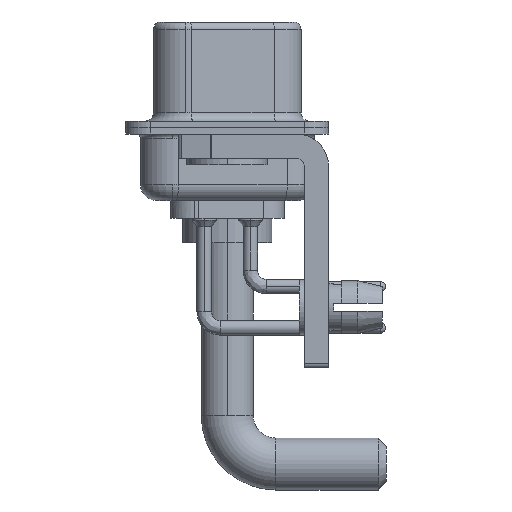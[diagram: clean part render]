
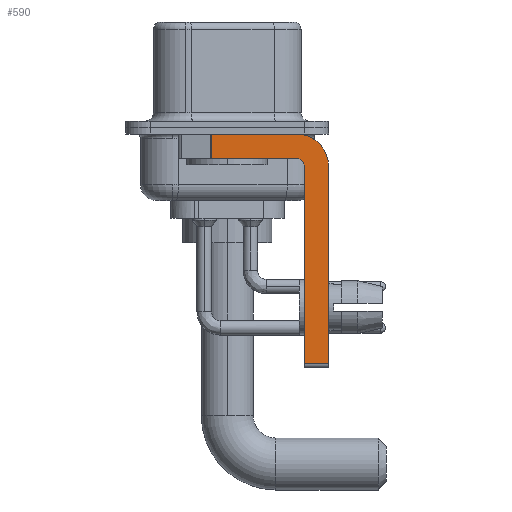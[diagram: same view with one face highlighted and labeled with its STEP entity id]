
A CAD part, left-side view. The second image highlights one B-rep face of the part: STEP entity #590.
In plain terms, the highlighted planar face has unit normal (-1, 0, 0).
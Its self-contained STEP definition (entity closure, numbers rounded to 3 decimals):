
#542 = VECTOR ( 'NONE', #23690, 1000. ) ;
#590 = ADVANCED_FACE ( 'NONE', ( #19994 ), #11389, .F. ) ;
#682 = VERTEX_POINT ( 'NONE', #23240 ) ;
#734 = LINE ( 'NONE', #13457, #12163 ) ;
#1258 = VERTEX_POINT ( 'NONE', #10749 ) ;
#1334 = ORIENTED_EDGE ( 'NONE', *, *, #7442, .T. ) ;
#1344 = VERTEX_POINT ( 'NONE', #19079 ) ;
#1639 = EDGE_CURVE ( 'NONE', #10639, #682, #2580, .T. ) ;
#1990 = DIRECTION ( 'NONE',  ( -1., 0., 0. ) ) ;
#2530 = CARTESIAN_POINT ( 'NONE',  ( -2.9, -4.25, -14.55 ) ) ;
#2580 = CIRCLE ( 'NONE', #28166, 0.5 ) ;
#2780 = CARTESIAN_POINT ( 'NONE',  ( -2.9, -4.75, -14.55 ) ) ;
#3087 = DIRECTION ( 'NONE',  ( 0., 0., -1. ) ) ;
#3308 = VECTOR ( 'NONE', #16369, 1000. ) ;
#3680 = CARTESIAN_POINT ( 'NONE',  ( -2.9, -4.25, -1.9 ) ) ;
#3988 = EDGE_CURVE ( 'NONE', #1344, #25224, #22690, .T. ) ;
#4282 = LINE ( 'NONE', #21493, #17298 ) ;
#4372 = VERTEX_POINT ( 'NONE', #2780 ) ;
#4803 = CARTESIAN_POINT ( 'NONE',  ( -2.9, 3., -0.4 ) ) ;
#5787 = CIRCLE ( 'NONE', #21787, 2. ) ;
#7180 = EDGE_CURVE ( 'NONE', #682, #1258, #21429, .T. ) ;
#7442 = EDGE_CURVE ( 'NONE', #1344, #1258, #11670, .T. ) ;
#9121 = DIRECTION ( 'NONE',  ( 0., -1., 0. ) ) ;
#9535 = LINE ( 'NONE', #2530, #22934 ) ;
#10587 = CARTESIAN_POINT ( 'NONE',  ( -2.9, -4.25, -2.4 ) ) ;
#10639 = VERTEX_POINT ( 'NONE', #20645 ) ;
#10749 = CARTESIAN_POINT ( 'NONE',  ( -2.9, 0.978, -1.9 ) ) ;
#10981 = EDGE_CURVE ( 'NONE', #4372, #15280, #9535, .T. ) ;
#11389 = PLANE ( 'NONE',  #14396 ) ;
#11574 = CARTESIAN_POINT ( 'NONE',  ( -2.9, -4.25, -2.4 ) ) ;
#11670 = LINE ( 'NONE', #27244, #3308 ) ;
#12163 = VECTOR ( 'NONE', #20488, 1000. ) ;
#13457 = CARTESIAN_POINT ( 'NONE',  ( -2.9, -6.25, -2.4 ) ) ;
#13655 = VECTOR ( 'NONE', #26689, 1000. ) ;
#14396 = AXIS2_PLACEMENT_3D ( 'NONE', #15812, #26562, #3087 ) ;
#15280 = VERTEX_POINT ( 'NONE', #27460 ) ;
#15756 = ORIENTED_EDGE ( 'NONE', *, *, #1639, .F. ) ;
#15812 = CARTESIAN_POINT ( 'NONE',  ( -2.9, -4.25, -2.4 ) ) ;
#16369 = DIRECTION ( 'NONE',  ( 0., 0., -1. ) ) ;
#16483 = EDGE_CURVE ( 'NONE', #27638, #15280, #734, .T. ) ;
#16925 = EDGE_CURVE ( 'NONE', #25224, #27638, #5787, .T. ) ;
#17298 = VECTOR ( 'NONE', #25756, 1000. ) ;
#17364 = EDGE_LOOP ( 'NONE', ( #22047, #1334, #21734, #15756, #26348, #23552, #20946, #27428 ) ) ;
#18822 = CARTESIAN_POINT ( 'NONE',  ( -2.9, -6.25, -2.4 ) ) ;
#19079 = CARTESIAN_POINT ( 'NONE',  ( -2.9, 0.978, -0.4 ) ) ;
#19994 = FACE_OUTER_BOUND ( 'NONE', #17364, .T. ) ;
#20488 = DIRECTION ( 'NONE',  ( 0., 0., -1. ) ) ;
#20645 = CARTESIAN_POINT ( 'NONE',  ( -2.9, -4.75, -2.4 ) ) ;
#20946 = ORIENTED_EDGE ( 'NONE', *, *, #16483, .F. ) ;
#21429 = LINE ( 'NONE', #3680, #542 ) ;
#21493 = CARTESIAN_POINT ( 'NONE',  ( -2.9, -4.75, -14.8 ) ) ;
#21734 = ORIENTED_EDGE ( 'NONE', *, *, #7180, .F. ) ;
#21787 = AXIS2_PLACEMENT_3D ( 'NONE', #11574, #22317, #22588 ) ;
#22047 = ORIENTED_EDGE ( 'NONE', *, *, #3988, .F. ) ;
#22317 = DIRECTION ( 'NONE',  ( 1., 0., 0. ) ) ;
#22588 = DIRECTION ( 'NONE',  ( 0., 0., -1. ) ) ;
#22690 = LINE ( 'NONE', #4803, #13655 ) ;
#22934 = VECTOR ( 'NONE', #9121, 1000. ) ;
#23240 = CARTESIAN_POINT ( 'NONE',  ( -2.9, -4.25, -1.9 ) ) ;
#23312 = DIRECTION ( 'NONE',  ( 0., 0., 1. ) ) ;
#23552 = ORIENTED_EDGE ( 'NONE', *, *, #10981, .T. ) ;
#23690 = DIRECTION ( 'NONE',  ( 0., 1., 0. ) ) ;
#25224 = VERTEX_POINT ( 'NONE', #26547 ) ;
#25756 = DIRECTION ( 'NONE',  ( 0., 0., 1. ) ) ;
#26348 = ORIENTED_EDGE ( 'NONE', *, *, #28149, .F. ) ;
#26547 = CARTESIAN_POINT ( 'NONE',  ( -2.9, -4.25, -0.4 ) ) ;
#26562 = DIRECTION ( 'NONE',  ( 1., 0., 0. ) ) ;
#26689 = DIRECTION ( 'NONE',  ( 0., -1., 0. ) ) ;
#27244 = CARTESIAN_POINT ( 'NONE',  ( -2.9, 0.978, -1.9 ) ) ;
#27428 = ORIENTED_EDGE ( 'NONE', *, *, #16925, .F. ) ;
#27460 = CARTESIAN_POINT ( 'NONE',  ( -2.9, -6.25, -14.55 ) ) ;
#27638 = VERTEX_POINT ( 'NONE', #18822 ) ;
#28149 = EDGE_CURVE ( 'NONE', #4372, #10639, #4282, .T. ) ;
#28166 = AXIS2_PLACEMENT_3D ( 'NONE', #10587, #1990, #23312 ) ;
